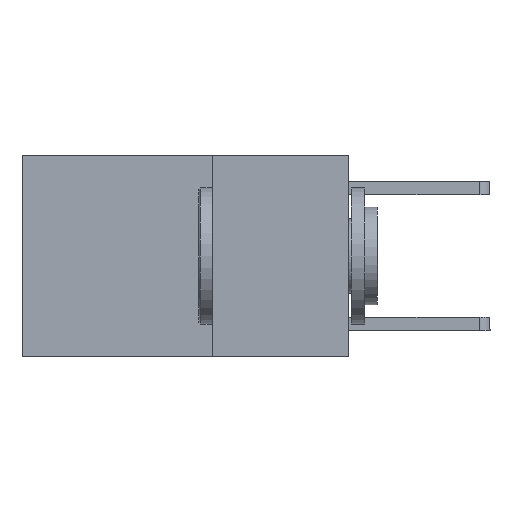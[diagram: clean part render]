
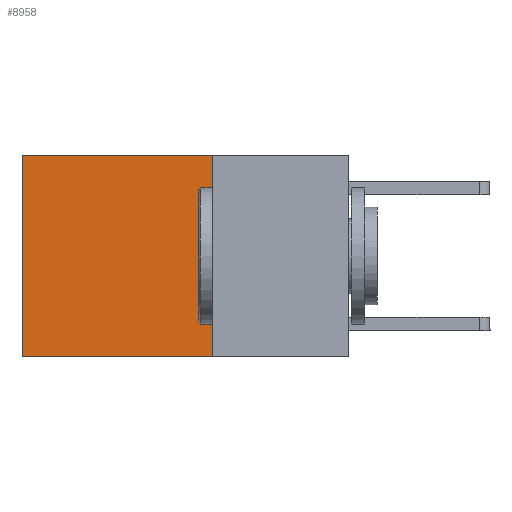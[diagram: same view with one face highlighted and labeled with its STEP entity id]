
A CAD part, left-side view. The second image highlights one B-rep face of the part: STEP entity #8958.
In plain terms, the highlighted planar face has unit normal (-1, 0, 0).
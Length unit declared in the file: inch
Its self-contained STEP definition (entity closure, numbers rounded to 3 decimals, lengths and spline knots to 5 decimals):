
#111 = ORIENTED_EDGE ( 'NONE', *, *, #1181, .F. ) ;
#205 = CARTESIAN_POINT ( 'NONE',  ( 0.2625, 0.6, 0. ) ) ;
#516 = DIRECTION ( 'NONE',  ( 0., 0., -1. ) ) ;
#522 = VERTEX_POINT ( 'NONE', #8793 ) ;
#753 = EDGE_CURVE ( 'NONE', #4245, #5056, #8204, .T. ) ;
#783 = AXIS2_PLACEMENT_3D ( 'NONE', #5951, #4481, #516 ) ;
#808 = ORIENTED_EDGE ( 'NONE', *, *, #753, .T. ) ;
#1181 = EDGE_CURVE ( 'NONE', #522, #3206, #9028, .T. ) ;
#1514 = CARTESIAN_POINT ( 'NONE',  ( 0.2625, 0.25, -0.37 ) ) ;
#1654 = ORIENTED_EDGE ( 'NONE', *, *, #4507, .F. ) ;
#2570 = CARTESIAN_POINT ( 'NONE',  ( 0.2625, 0.25, 0. ) ) ;
#2763 = VECTOR ( 'NONE', #9270, 39.37008 ) ;
#2766 = FACE_OUTER_BOUND ( 'NONE', #6747, .T. ) ;
#2840 = CARTESIAN_POINT ( 'NONE',  ( 0.2625, 0.6, 0. ) ) ;
#3052 = VECTOR ( 'NONE', #6022, 39.37008 ) ;
#3206 = VERTEX_POINT ( 'NONE', #1514 ) ;
#3476 = CARTESIAN_POINT ( 'NONE',  ( 0.2625, 0.6, -0.37 ) ) ;
#3893 = ORIENTED_EDGE ( 'NONE', *, *, #5280, .T. ) ;
#4245 = VERTEX_POINT ( 'NONE', #205 ) ;
#4481 = DIRECTION ( 'NONE',  ( 1., 0., 0. ) ) ;
#4507 = EDGE_CURVE ( 'NONE', #3206, #5056, #9429, .T. ) ;
#5056 = VERTEX_POINT ( 'NONE', #3476 ) ;
#5280 = EDGE_CURVE ( 'NONE', #522, #4245, #7964, .T. ) ;
#5907 = DIRECTION ( 'NONE',  ( 0., 0., -1. ) ) ;
#5951 = CARTESIAN_POINT ( 'NONE',  ( 0.2625, 0.25, 0. ) ) ;
#6022 = DIRECTION ( 'NONE',  ( 0., 0., -1. ) ) ;
#6158 = CARTESIAN_POINT ( 'NONE',  ( 0.2625, 0.25, -0.37 ) ) ;
#6747 = EDGE_LOOP ( 'NONE', ( #808, #1654, #111, #3893 ) ) ;
#7162 = VECTOR ( 'NONE', #5907, 39.37008 ) ;
#7171 = DIRECTION ( 'NONE',  ( 0., 1., 0. ) ) ;
#7659 = PLANE ( 'NONE',  #783 ) ;
#7964 = LINE ( 'NONE', #8530, #8422 ) ;
#8204 = LINE ( 'NONE', #2840, #3052 ) ;
#8422 = VECTOR ( 'NONE', #7171, 39.37008 ) ;
#8530 = CARTESIAN_POINT ( 'NONE',  ( 0.2625, 0.25, 0. ) ) ;
#8793 = CARTESIAN_POINT ( 'NONE',  ( 0.2625, 0.25, 0. ) ) ;
#8958 = ADVANCED_FACE ( 'NONE', ( #2766 ), #7659, .F. ) ;
#9028 = LINE ( 'NONE', #2570, #7162 ) ;
#9270 = DIRECTION ( 'NONE',  ( 0., 1., 0. ) ) ;
#9429 = LINE ( 'NONE', #6158, #2763 ) ;
